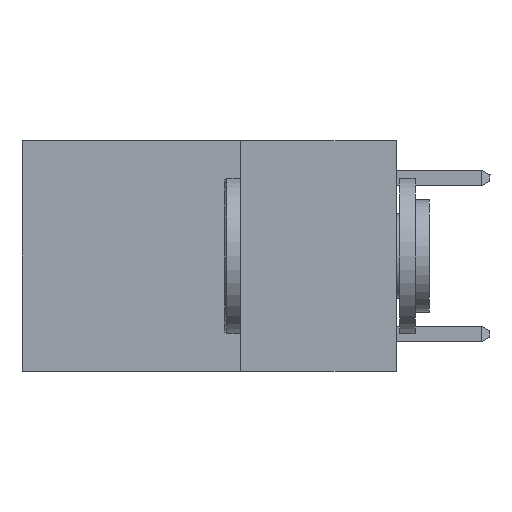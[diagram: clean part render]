
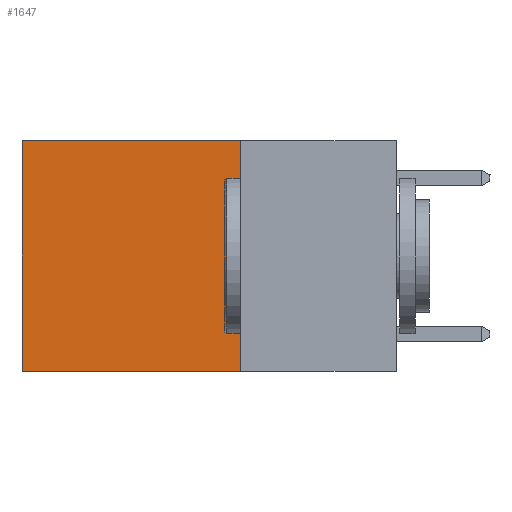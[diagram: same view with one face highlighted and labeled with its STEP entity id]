
A CAD part, left-side view. The second image highlights one B-rep face of the part: STEP entity #1647.
In plain terms, the highlighted planar face has unit normal (-1, 0, 0).
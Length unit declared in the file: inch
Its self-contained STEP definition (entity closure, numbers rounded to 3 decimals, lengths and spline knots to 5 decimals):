
#233 = ORIENTED_EDGE ( 'NONE', *, *, #13461, .F. ) ;
#1647 = ADVANCED_FACE ( 'NONE', ( #21947 ), #26756, .F. ) ;
#1887 = CARTESIAN_POINT ( 'NONE',  ( 0.2625, 0.6, 0. ) ) ;
#2332 = CARTESIAN_POINT ( 'NONE',  ( 0.2625, 0.25, -0.37 ) ) ;
#3674 = EDGE_CURVE ( 'NONE', #7534, #14806, #31229, .T. ) ;
#4094 = DIRECTION ( 'NONE',  ( 0., 0., -1. ) ) ;
#4695 = CARTESIAN_POINT ( 'NONE',  ( 0.2625, 0.6, -0.37 ) ) ;
#4795 = DIRECTION ( 'NONE',  ( 0., 0., -1. ) ) ;
#5277 = CARTESIAN_POINT ( 'NONE',  ( 0.2625, 0.25, 0. ) ) ;
#6493 = LINE ( 'NONE', #16304, #27127 ) ;
#6866 = DIRECTION ( 'NONE',  ( 0., 1., 0. ) ) ;
#7534 = VERTEX_POINT ( 'NONE', #5277 ) ;
#8424 = LINE ( 'NONE', #18236, #21450 ) ;
#9588 = EDGE_CURVE ( 'NONE', #14806, #13916, #8424, .T. ) ;
#10913 = AXIS2_PLACEMENT_3D ( 'NONE', #12483, #22422, #4795 ) ;
#11983 = VECTOR ( 'NONE', #26617, 39.37008 ) ;
#12483 = CARTESIAN_POINT ( 'NONE',  ( 0.2625, 0.25, 0. ) ) ;
#13461 = EDGE_CURVE ( 'NONE', #7534, #30415, #6493, .T. ) ;
#13916 = VERTEX_POINT ( 'NONE', #4695 ) ;
#14604 = LINE ( 'NONE', #14761, #11983 ) ;
#14761 = CARTESIAN_POINT ( 'NONE',  ( 0.2625, 0.25, -0.37 ) ) ;
#14806 = VERTEX_POINT ( 'NONE', #1887 ) ;
#16304 = CARTESIAN_POINT ( 'NONE',  ( 0.2625, 0.25, 0. ) ) ;
#16841 = ORIENTED_EDGE ( 'NONE', *, *, #3674, .T. ) ;
#18167 = ORIENTED_EDGE ( 'NONE', *, *, #9588, .T. ) ;
#18236 = CARTESIAN_POINT ( 'NONE',  ( 0.2625, 0.6, 0. ) ) ;
#19091 = CARTESIAN_POINT ( 'NONE',  ( 0.2625, 0.25, 0. ) ) ;
#19275 = ORIENTED_EDGE ( 'NONE', *, *, #28108, .F. ) ;
#20470 = DIRECTION ( 'NONE',  ( 0., 0., -1. ) ) ;
#21450 = VECTOR ( 'NONE', #20470, 39.37008 ) ;
#21947 = FACE_OUTER_BOUND ( 'NONE', #27577, .T. ) ;
#22422 = DIRECTION ( 'NONE',  ( 1., 0., 0. ) ) ;
#26617 = DIRECTION ( 'NONE',  ( 0., 1., 0. ) ) ;
#26756 = PLANE ( 'NONE',  #10913 ) ;
#27127 = VECTOR ( 'NONE', #4094, 39.37008 ) ;
#27577 = EDGE_LOOP ( 'NONE', ( #18167, #19275, #233, #16841 ) ) ;
#28108 = EDGE_CURVE ( 'NONE', #30415, #13916, #14604, .T. ) ;
#29543 = VECTOR ( 'NONE', #6866, 39.37008 ) ;
#30415 = VERTEX_POINT ( 'NONE', #2332 ) ;
#31229 = LINE ( 'NONE', #19091, #29543 ) ;
